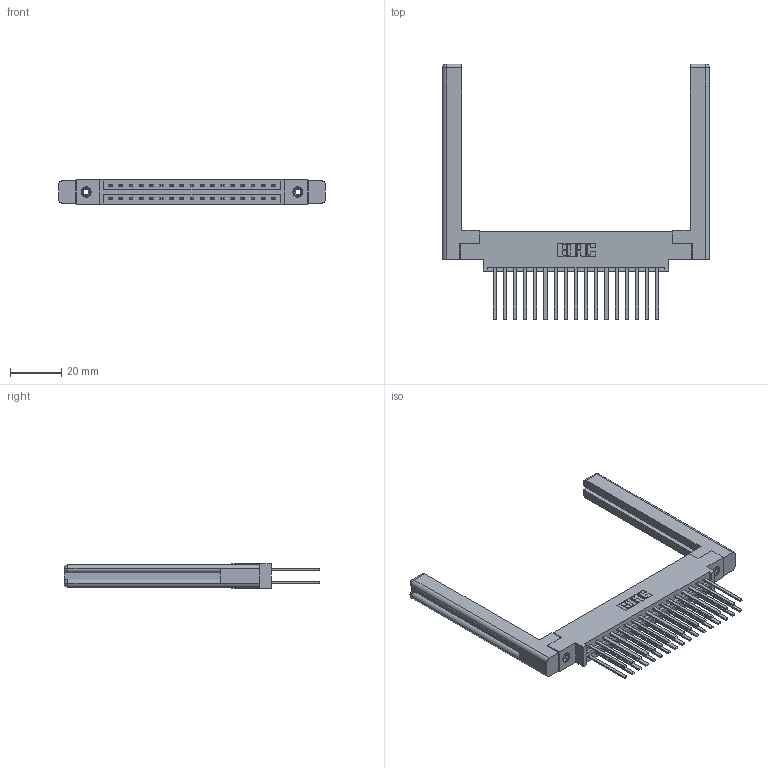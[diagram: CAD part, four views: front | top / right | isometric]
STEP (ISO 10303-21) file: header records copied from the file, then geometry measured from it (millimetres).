
FILE_DESCRIPTION (( 'STEP AP203' ), '1' );
FILE_NAME ('387-034-544-858.STEP', '2019-10-17T17:52:10', ( '' ), ( '' ), 'SwSTEP 2.0', 'SolidWorks 2016', '' );
FILE_SCHEMA (( 'CONFIG_CONTROL_DESIGN' ));
Length unit declared in the file: inch
Products named in the file (5): 387-034-544-858; 307-220-058; 337 Part_0.170 Offset - 0.156 Dia-TI; 345-250-001_345-250-001-102; 345-292-001_345-293-144
Assembly tree (39 placements, depth 2):
  387-034-544-858
    337 Part_0.170 Offset - 0.156 Dia-TI
    345-292-001_345-293-144  x34
    345-250-001_345-250-001-102  x2
    307-220-058  x2
Bounding box: 103.99 x 99.7 x 9.4 mm (x, y, z)
Volume: 18127.7 mm3; surface area: 18887.7 mm2
Topology: 39 solids, 39 shells, 1892 faces, 5539 edges, 3634 vertices
Faces by surface type: plane 1314, cylinder 554, cone 12, torus 12
Entity records: 18996 total; most frequent: CARTESIAN_POINT 3229, ORIENTED_EDGE 3104, DIRECTION 2804, EDGE_CURVE 1552, LINE 1380, VECTOR 1380, VERTEX_POINT 1026, AXIS2_PLACEMENT_3D 712
